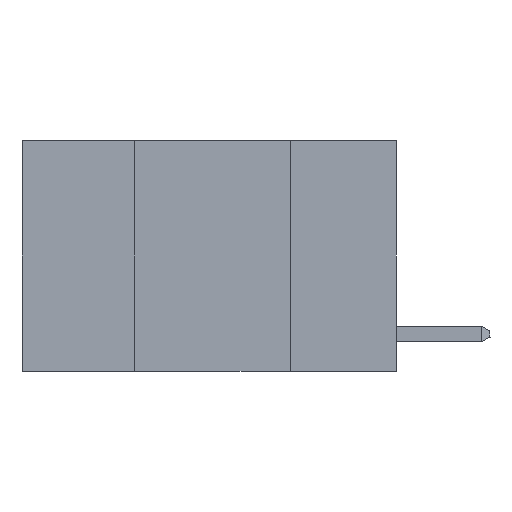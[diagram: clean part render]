
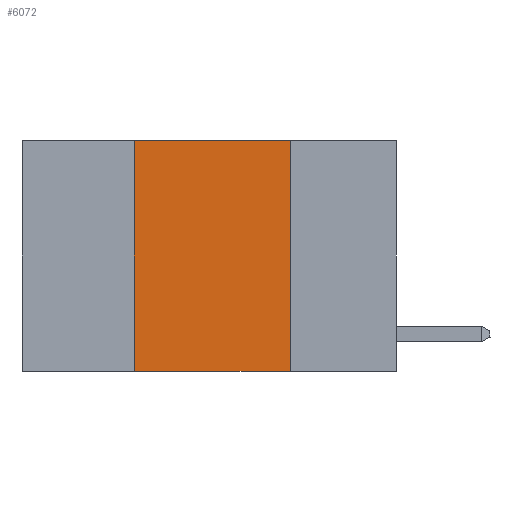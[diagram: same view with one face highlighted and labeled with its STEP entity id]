
A CAD part, left-side view. The second image highlights one B-rep face of the part: STEP entity #6072.
In plain terms, the highlighted planar face has unit normal (-1, 0, 0).
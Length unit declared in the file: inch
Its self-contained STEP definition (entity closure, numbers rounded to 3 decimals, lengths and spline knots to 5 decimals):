
#677 = DIRECTION ( 'NONE',  ( 0., -1., 0. ) ) ;
#1529 = DIRECTION ( 'NONE',  ( 0., 0., 1. ) ) ;
#1984 = CARTESIAN_POINT ( 'NONE',  ( 0., 0.17, 0. ) ) ;
#2103 = EDGE_LOOP ( 'NONE', ( #4319, #15102, #22021, #14723 ) ) ;
#2173 = CARTESIAN_POINT ( 'NONE',  ( 0., 0.42, -0.37 ) ) ;
#2571 = LINE ( 'NONE', #18972, #14570 ) ;
#4319 = ORIENTED_EDGE ( 'NONE', *, *, #15386, .F. ) ;
#4829 = CARTESIAN_POINT ( 'NONE',  ( 0., 0.42, 0. ) ) ;
#5695 = CARTESIAN_POINT ( 'NONE',  ( 0., 0.6, 0. ) ) ;
#5728 = VECTOR ( 'NONE', #677, 39.37008 ) ;
#6072 = ADVANCED_FACE ( 'NONE', ( #19856 ), #14479, .F. ) ;
#7348 = VERTEX_POINT ( 'NONE', #22585 ) ;
#7666 = VERTEX_POINT ( 'NONE', #1984 ) ;
#8365 = VECTOR ( 'NONE', #1529, 39.37008 ) ;
#8711 = EDGE_CURVE ( 'NONE', #9123, #18801, #9004, .T. ) ;
#8853 = EDGE_CURVE ( 'NONE', #18801, #7666, #20539, .T. ) ;
#9004 = LINE ( 'NONE', #19837, #8365 ) ;
#9123 = VERTEX_POINT ( 'NONE', #2173 ) ;
#9471 = CARTESIAN_POINT ( 'NONE',  ( 0., 0.6, 0. ) ) ;
#9898 = DIRECTION ( 'NONE',  ( 0., 0., -1. ) ) ;
#11667 = CARTESIAN_POINT ( 'NONE',  ( 0., 0.17, 0. ) ) ;
#13688 = LINE ( 'NONE', #11667, #17822 ) ;
#13995 = AXIS2_PLACEMENT_3D ( 'NONE', #5695, #23429, #14829 ) ;
#14479 = PLANE ( 'NONE',  #13995 ) ;
#14570 = VECTOR ( 'NONE', #15149, 39.37008 ) ;
#14723 = ORIENTED_EDGE ( 'NONE', *, *, #20504, .T. ) ;
#14829 = DIRECTION ( 'NONE',  ( 0., 0., -1. ) ) ;
#15102 = ORIENTED_EDGE ( 'NONE', *, *, #8853, .F. ) ;
#15149 = DIRECTION ( 'NONE',  ( 0., -1., 0. ) ) ;
#15386 = EDGE_CURVE ( 'NONE', #7666, #7348, #13688, .T. ) ;
#17822 = VECTOR ( 'NONE', #9898, 39.37008 ) ;
#18801 = VERTEX_POINT ( 'NONE', #4829 ) ;
#18972 = CARTESIAN_POINT ( 'NONE',  ( 0., 0.6, -0.37 ) ) ;
#19837 = CARTESIAN_POINT ( 'NONE',  ( 0., 0.42, 0. ) ) ;
#19856 = FACE_OUTER_BOUND ( 'NONE', #2103, .T. ) ;
#20504 = EDGE_CURVE ( 'NONE', #9123, #7348, #2571, .T. ) ;
#20539 = LINE ( 'NONE', #9471, #5728 ) ;
#22021 = ORIENTED_EDGE ( 'NONE', *, *, #8711, .F. ) ;
#22585 = CARTESIAN_POINT ( 'NONE',  ( 0., 0.17, -0.37 ) ) ;
#23429 = DIRECTION ( 'NONE',  ( 1., 0., 0. ) ) ;
